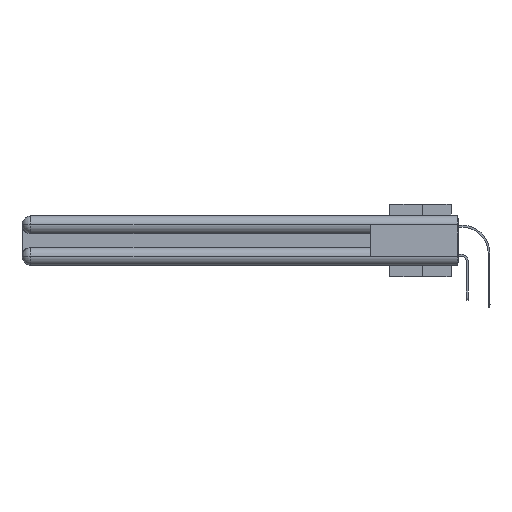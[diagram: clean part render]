
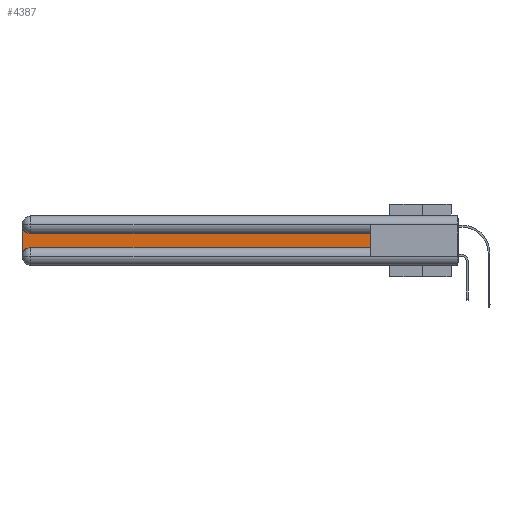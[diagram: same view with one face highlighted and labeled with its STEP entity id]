
A CAD part, left-side view. The second image highlights one B-rep face of the part: STEP entity #4387.
In plain terms, the highlighted planar face has unit normal (-1, 0, 0).
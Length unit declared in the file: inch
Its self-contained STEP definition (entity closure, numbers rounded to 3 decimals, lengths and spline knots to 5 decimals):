
#809 = CIRCLE ( 'NONE', #9870, 0.06 ) ;
#857 = ORIENTED_EDGE ( 'NONE', *, *, #3786, .T. ) ;
#1364 = LINE ( 'NONE', #4644, #41260 ) ;
#1925 = DIRECTION ( 'NONE',  ( 1., 0., 0. ) ) ;
#2289 = LINE ( 'NONE', #17985, #15374 ) ;
#2426 = DIRECTION ( 'NONE',  ( 0., 0., 1. ) ) ;
#2632 = CARTESIAN_POINT ( 'NONE',  ( 0.075, 0.6, -0.2175 ) ) ;
#2957 = CIRCLE ( 'NONE', #8542, 0.06 ) ;
#3203 = ORIENTED_EDGE ( 'NONE', *, *, #6485, .T. ) ;
#3786 = EDGE_CURVE ( 'NONE', #8352, #19611, #30732, .T. ) ;
#4387 = ADVANCED_FACE ( 'NONE', ( #15000 ), #18908, .F. ) ;
#4481 = ORIENTED_EDGE ( 'NONE', *, *, #10021, .T. ) ;
#4644 = CARTESIAN_POINT ( 'NONE',  ( 0.075, 3., -0.2175 ) ) ;
#5099 = ORIENTED_EDGE ( 'NONE', *, *, #23406, .T. ) ;
#5347 = CARTESIAN_POINT ( 'NONE',  ( 0.075, 0.6, -0.1225 ) ) ;
#6485 = EDGE_CURVE ( 'NONE', #19611, #23368, #28739, .T. ) ;
#8235 = VERTEX_POINT ( 'NONE', #11608 ) ;
#8352 = VERTEX_POINT ( 'NONE', #12243 ) ;
#8542 = AXIS2_PLACEMENT_3D ( 'NONE', #40227, #33048, #13283 ) ;
#9293 = EDGE_CURVE ( 'NONE', #8235, #28248, #1364, .T. ) ;
#9870 = AXIS2_PLACEMENT_3D ( 'NONE', #35739, #12481, #38795 ) ;
#10021 = EDGE_CURVE ( 'NONE', #28248, #8352, #2957, .T. ) ;
#11608 = CARTESIAN_POINT ( 'NONE',  ( 0.075, 3., -0.0625 ) ) ;
#12243 = CARTESIAN_POINT ( 'NONE',  ( 0.075, 2.94, -0.2175 ) ) ;
#12481 = DIRECTION ( 'NONE',  ( 1., 0., 0. ) ) ;
#13283 = DIRECTION ( 'NONE',  ( 0., 0., -1. ) ) ;
#15000 = FACE_OUTER_BOUND ( 'NONE', #17194, .T. ) ;
#15374 = VECTOR ( 'NONE', #38632, 39.37008 ) ;
#17194 = EDGE_LOOP ( 'NONE', ( #5099, #25638, #37686, #4481, #857, #3203 ) ) ;
#17985 = CARTESIAN_POINT ( 'NONE',  ( 0.075, 0.6, -0.1225 ) ) ;
#18786 = VECTOR ( 'NONE', #2426, 39.37008 ) ;
#18908 = PLANE ( 'NONE',  #27884 ) ;
#19133 = DIRECTION ( 'NONE',  ( 0., 0., -1. ) ) ;
#19611 = VERTEX_POINT ( 'NONE', #20549 ) ;
#20549 = CARTESIAN_POINT ( 'NONE',  ( 0.075, 0.6, -0.2175 ) ) ;
#21500 = VERTEX_POINT ( 'NONE', #28478 ) ;
#21957 = CARTESIAN_POINT ( 'NONE',  ( 0.075, 3., -0.2775 ) ) ;
#23368 = VERTEX_POINT ( 'NONE', #5347 ) ;
#23373 = DIRECTION ( 'NONE',  ( 0., -1., 0. ) ) ;
#23406 = EDGE_CURVE ( 'NONE', #23368, #21500, #2289, .T. ) ;
#24981 = CARTESIAN_POINT ( 'NONE',  ( 0.075, 3., -0.1225 ) ) ;
#25085 = DIRECTION ( 'NONE',  ( 0., 0., -1. ) ) ;
#25638 = ORIENTED_EDGE ( 'NONE', *, *, #30358, .T. ) ;
#27489 = CARTESIAN_POINT ( 'NONE',  ( 0.075, 0.6, -0.2175 ) ) ;
#27884 = AXIS2_PLACEMENT_3D ( 'NONE', #24981, #1925, #19133 ) ;
#28248 = VERTEX_POINT ( 'NONE', #21957 ) ;
#28478 = CARTESIAN_POINT ( 'NONE',  ( 0.075, 2.94, -0.1225 ) ) ;
#28739 = LINE ( 'NONE', #2632, #18786 ) ;
#30358 = EDGE_CURVE ( 'NONE', #21500, #8235, #809, .T. ) ;
#30732 = LINE ( 'NONE', #27489, #31187 ) ;
#31187 = VECTOR ( 'NONE', #23373, 39.37008 ) ;
#33048 = DIRECTION ( 'NONE',  ( 1., 0., 0. ) ) ;
#35739 = CARTESIAN_POINT ( 'NONE',  ( 0.075, 2.94, -0.0625 ) ) ;
#37686 = ORIENTED_EDGE ( 'NONE', *, *, #9293, .T. ) ;
#38632 = DIRECTION ( 'NONE',  ( 0., 1., 0. ) ) ;
#38795 = DIRECTION ( 'NONE',  ( 0., 0., -1. ) ) ;
#40227 = CARTESIAN_POINT ( 'NONE',  ( 0.075, 2.94, -0.2775 ) ) ;
#41260 = VECTOR ( 'NONE', #25085, 39.37008 ) ;
